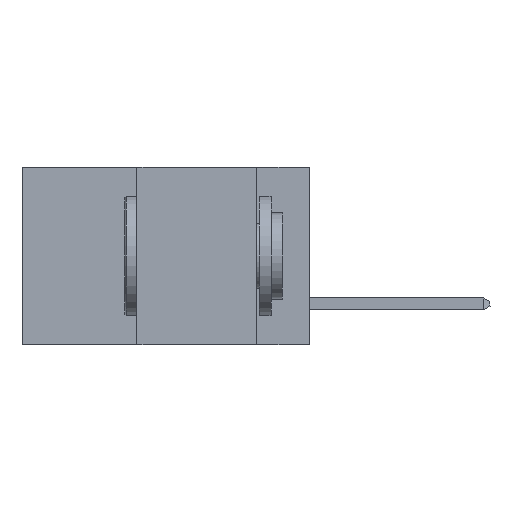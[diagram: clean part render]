
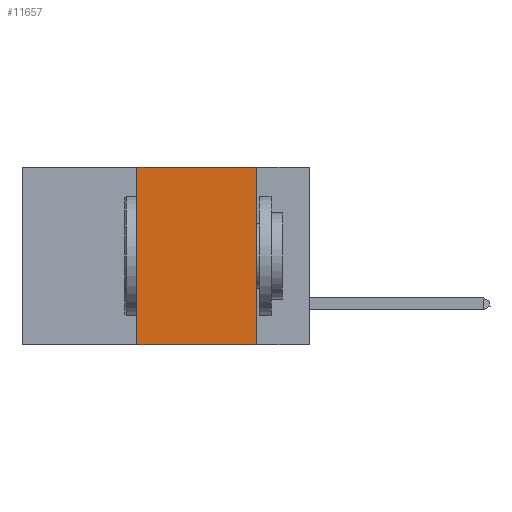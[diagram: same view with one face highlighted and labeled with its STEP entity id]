
A CAD part, left-side view. The second image highlights one B-rep face of the part: STEP entity #11657.
In plain terms, the highlighted planar face has unit normal (-1, 0, 0).
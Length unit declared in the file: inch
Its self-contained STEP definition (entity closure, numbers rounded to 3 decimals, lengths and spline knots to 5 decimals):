
#1156 = CARTESIAN_POINT ( 'NONE',  ( 0., 0.6, 0. ) ) ;
#2641 = VERTEX_POINT ( 'NONE', #7990 ) ;
#2672 = FACE_OUTER_BOUND ( 'NONE', #25621, .T. ) ;
#3114 = VERTEX_POINT ( 'NONE', #22802 ) ;
#3430 = DIRECTION ( 'NONE',  ( 1., 0., 0. ) ) ;
#4285 = AXIS2_PLACEMENT_3D ( 'NONE', #1156, #3430, #18979 ) ;
#5223 = EDGE_CURVE ( 'NONE', #9130, #10116, #26978, .T. ) ;
#5305 = ORIENTED_EDGE ( 'NONE', *, *, #14001, .F. ) ;
#6314 = CARTESIAN_POINT ( 'NONE',  ( 0., 0.36, -0.37 ) ) ;
#6738 = EDGE_CURVE ( 'NONE', #9130, #3114, #16961, .T. ) ;
#7060 = ORIENTED_EDGE ( 'NONE', *, *, #5223, .T. ) ;
#7990 = CARTESIAN_POINT ( 'NONE',  ( 0., 0.11, 0. ) ) ;
#8223 = EDGE_CURVE ( 'NONE', #2641, #10116, #12309, .T. ) ;
#8251 = DIRECTION ( 'NONE',  ( 0., -1., 0. ) ) ;
#9130 = VERTEX_POINT ( 'NONE', #6314 ) ;
#10071 = VECTOR ( 'NONE', #18573, 39.37008 ) ;
#10116 = VERTEX_POINT ( 'NONE', #18457 ) ;
#11292 = DIRECTION ( 'NONE',  ( 0., 0., 1. ) ) ;
#11657 = ADVANCED_FACE ( 'NONE', ( #2672 ), #14549, .F. ) ;
#11814 = VECTOR ( 'NONE', #11292, 39.37008 ) ;
#12309 = LINE ( 'NONE', #18927, #18161 ) ;
#13346 = ORIENTED_EDGE ( 'NONE', *, *, #8223, .F. ) ;
#14001 = EDGE_CURVE ( 'NONE', #3114, #2641, #21741, .T. ) ;
#14153 = CARTESIAN_POINT ( 'NONE',  ( 0., 0.6, 0. ) ) ;
#14507 = DIRECTION ( 'NONE',  ( 0., 0., -1. ) ) ;
#14549 = PLANE ( 'NONE',  #4285 ) ;
#16961 = LINE ( 'NONE', #22218, #11814 ) ;
#18161 = VECTOR ( 'NONE', #14507, 39.37008 ) ;
#18457 = CARTESIAN_POINT ( 'NONE',  ( 0., 0.11, -0.37 ) ) ;
#18573 = DIRECTION ( 'NONE',  ( 0., -1., 0. ) ) ;
#18927 = CARTESIAN_POINT ( 'NONE',  ( 0., 0.11, 0. ) ) ;
#18979 = DIRECTION ( 'NONE',  ( 0., 0., -1. ) ) ;
#19261 = CARTESIAN_POINT ( 'NONE',  ( 0., 0.6, -0.37 ) ) ;
#19514 = ORIENTED_EDGE ( 'NONE', *, *, #6738, .F. ) ;
#21741 = LINE ( 'NONE', #14153, #10071 ) ;
#21846 = VECTOR ( 'NONE', #8251, 39.37008 ) ;
#22218 = CARTESIAN_POINT ( 'NONE',  ( 0., 0.36, 0. ) ) ;
#22802 = CARTESIAN_POINT ( 'NONE',  ( 0., 0.36, 0. ) ) ;
#25621 = EDGE_LOOP ( 'NONE', ( #13346, #5305, #19514, #7060 ) ) ;
#26978 = LINE ( 'NONE', #19261, #21846 ) ;
